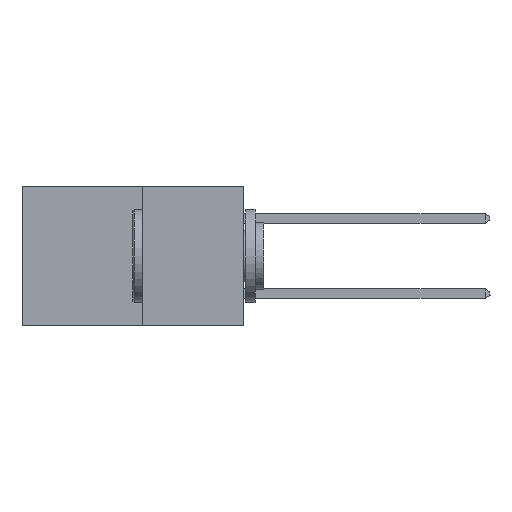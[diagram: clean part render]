
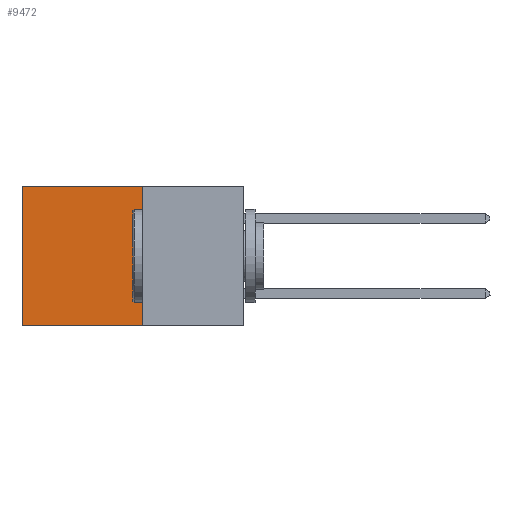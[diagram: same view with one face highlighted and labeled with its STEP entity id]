
A CAD part, left-side view. The second image highlights one B-rep face of the part: STEP entity #9472.
In plain terms, the highlighted planar face has unit normal (-1, 0, 0).
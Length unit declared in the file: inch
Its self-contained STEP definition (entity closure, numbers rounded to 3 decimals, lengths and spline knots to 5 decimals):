
#522 = LINE ( 'NONE', #24823, #24051 ) ;
#2592 = FACE_OUTER_BOUND ( 'NONE', #6198, .T. ) ;
#3377 = EDGE_CURVE ( 'NONE', #24760, #10486, #13881, .T. ) ;
#4089 = LINE ( 'NONE', #25505, #21000 ) ;
#5699 = CARTESIAN_POINT ( 'NONE',  ( 0.277, 0.59, 0. ) ) ;
#6198 = EDGE_LOOP ( 'NONE', ( #10233, #11872, #10808, #9928 ) ) ;
#6452 = EDGE_CURVE ( 'NONE', #18520, #21207, #4089, .T. ) ;
#8726 = VECTOR ( 'NONE', #14194, 39.37008 ) ;
#9122 = EDGE_CURVE ( 'NONE', #10486, #21207, #522, .T. ) ;
#9472 = ADVANCED_FACE ( 'NONE', ( #2592 ), #20161, .F. ) ;
#9928 = ORIENTED_EDGE ( 'NONE', *, *, #3377, .T. ) ;
#10233 = ORIENTED_EDGE ( 'NONE', *, *, #9122, .T. ) ;
#10486 = VERTEX_POINT ( 'NONE', #5699 ) ;
#10808 = ORIENTED_EDGE ( 'NONE', *, *, #12246, .F. ) ;
#11872 = ORIENTED_EDGE ( 'NONE', *, *, #6452, .F. ) ;
#12246 = EDGE_CURVE ( 'NONE', #24760, #18520, #13808, .T. ) ;
#12981 = CARTESIAN_POINT ( 'NONE',  ( 0.277, 0.27, -0.37 ) ) ;
#13299 = AXIS2_PLACEMENT_3D ( 'NONE', #19723, #19718, #19630 ) ;
#13703 = CARTESIAN_POINT ( 'NONE',  ( 0.277, 0.27, 0. ) ) ;
#13808 = LINE ( 'NONE', #18497, #19023 ) ;
#13881 = LINE ( 'NONE', #14269, #8726 ) ;
#14194 = DIRECTION ( 'NONE',  ( 0., 1., 0. ) ) ;
#14269 = CARTESIAN_POINT ( 'NONE',  ( 0.277, 0.27, 0. ) ) ;
#16372 = DIRECTION ( 'NONE',  ( 0., 0., -1. ) ) ;
#18497 = CARTESIAN_POINT ( 'NONE',  ( 0.277, 0.27, -0.37 ) ) ;
#18520 = VERTEX_POINT ( 'NONE', #12981 ) ;
#19023 = VECTOR ( 'NONE', #16372, 39.37008 ) ;
#19630 = DIRECTION ( 'NONE',  ( 0., 0., -1. ) ) ;
#19718 = DIRECTION ( 'NONE',  ( 1., 0., 0. ) ) ;
#19723 = CARTESIAN_POINT ( 'NONE',  ( 0.277, 0.27, -0.37 ) ) ;
#20161 = PLANE ( 'NONE',  #13299 ) ;
#20269 = CARTESIAN_POINT ( 'NONE',  ( 0.277, 0.59, -0.37 ) ) ;
#21000 = VECTOR ( 'NONE', #24968, 39.37008 ) ;
#21207 = VERTEX_POINT ( 'NONE', #20269 ) ;
#24051 = VECTOR ( 'NONE', #24764, 39.37008 ) ;
#24760 = VERTEX_POINT ( 'NONE', #13703 ) ;
#24764 = DIRECTION ( 'NONE',  ( 0., 0., -1. ) ) ;
#24823 = CARTESIAN_POINT ( 'NONE',  ( 0.277, 0.59, -0.37 ) ) ;
#24968 = DIRECTION ( 'NONE',  ( 0., 1., 0. ) ) ;
#25505 = CARTESIAN_POINT ( 'NONE',  ( 0.277, 0.27, -0.37 ) ) ;
